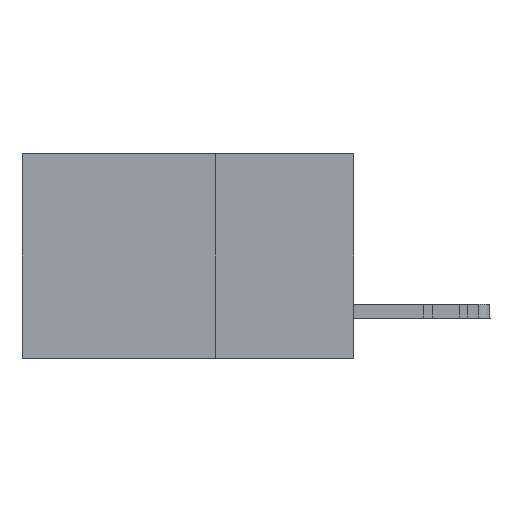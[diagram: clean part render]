
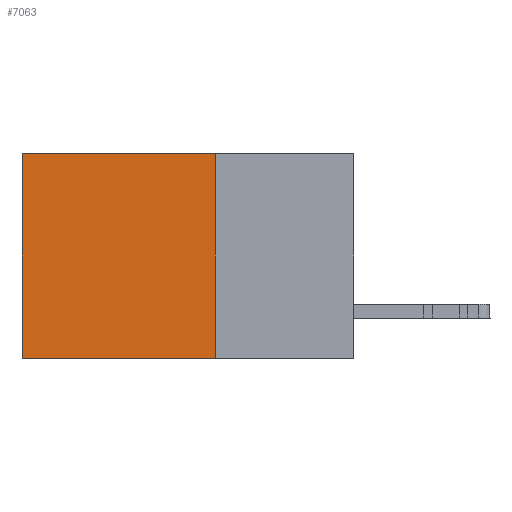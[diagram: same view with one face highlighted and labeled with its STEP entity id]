
A CAD part, left-side view. The second image highlights one B-rep face of the part: STEP entity #7063.
In plain terms, the highlighted planar face has unit normal (-1, 0, 0).
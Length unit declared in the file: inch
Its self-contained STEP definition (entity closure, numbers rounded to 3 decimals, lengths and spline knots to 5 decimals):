
#70 = CARTESIAN_POINT ( 'NONE',  ( 0.2875, 0.6, -0.37 ) ) ;
#145 = CARTESIAN_POINT ( 'NONE',  ( 0.2875, 0.25, 0. ) ) ;
#1344 = CARTESIAN_POINT ( 'NONE',  ( 0.2875, 0.25, 0. ) ) ;
#1549 = DIRECTION ( 'NONE',  ( 0., 0., -1. ) ) ;
#2447 = DIRECTION ( 'NONE',  ( 0., 0., -1. ) ) ;
#2676 = CARTESIAN_POINT ( 'NONE',  ( 0.2875, 0.6, 0. ) ) ;
#4258 = DIRECTION ( 'NONE',  ( 0., 0., -1. ) ) ;
#4470 = PLANE ( 'NONE',  #40602 ) ;
#6711 = LINE ( 'NONE', #6928, #41067 ) ;
#6928 = CARTESIAN_POINT ( 'NONE',  ( 0.2875, 0.25, 0. ) ) ;
#7063 = ADVANCED_FACE ( 'NONE', ( #8210 ), #4470, .F. ) ;
#8210 = FACE_OUTER_BOUND ( 'NONE', #25877, .T. ) ;
#8899 = VERTEX_POINT ( 'NONE', #20133 ) ;
#9793 = VERTEX_POINT ( 'NONE', #145 ) ;
#14824 = VECTOR ( 'NONE', #1549, 39.37008 ) ;
#16858 = CARTESIAN_POINT ( 'NONE',  ( 0.2875, 0.6, 0. ) ) ;
#20133 = CARTESIAN_POINT ( 'NONE',  ( 0.2875, 0.25, -0.37 ) ) ;
#20436 = VERTEX_POINT ( 'NONE', #70 ) ;
#20597 = VECTOR ( 'NONE', #25944, 39.37008 ) ;
#20605 = ORIENTED_EDGE ( 'NONE', *, *, #27931, .F. ) ;
#21529 = CARTESIAN_POINT ( 'NONE',  ( 0.2875, 0.25, 0. ) ) ;
#22233 = LINE ( 'NONE', #22448, #20597 ) ;
#22448 = CARTESIAN_POINT ( 'NONE',  ( 0.2875, 0.25, -0.37 ) ) ;
#23323 = VERTEX_POINT ( 'NONE', #16858 ) ;
#23448 = VECTOR ( 'NONE', #2447, 39.37008 ) ;
#23739 = DIRECTION ( 'NONE',  ( 0., 1., 0. ) ) ;
#25628 = LINE ( 'NONE', #2676, #23448 ) ;
#25678 = ORIENTED_EDGE ( 'NONE', *, *, #28863, .T. ) ;
#25877 = EDGE_LOOP ( 'NONE', ( #25678, #20605, #38654, #35409 ) ) ;
#25944 = DIRECTION ( 'NONE',  ( 0., 1., 0. ) ) ;
#27931 = EDGE_CURVE ( 'NONE', #8899, #20436, #22233, .T. ) ;
#28863 = EDGE_CURVE ( 'NONE', #23323, #20436, #25628, .T. ) ;
#31166 = DIRECTION ( 'NONE',  ( 1., 0., 0. ) ) ;
#33286 = EDGE_CURVE ( 'NONE', #9793, #23323, #6711, .T. ) ;
#35215 = LINE ( 'NONE', #1344, #14824 ) ;
#35409 = ORIENTED_EDGE ( 'NONE', *, *, #33286, .T. ) ;
#35872 = EDGE_CURVE ( 'NONE', #9793, #8899, #35215, .T. ) ;
#38654 = ORIENTED_EDGE ( 'NONE', *, *, #35872, .F. ) ;
#40602 = AXIS2_PLACEMENT_3D ( 'NONE', #21529, #31166, #4258 ) ;
#41067 = VECTOR ( 'NONE', #23739, 39.37008 ) ;
